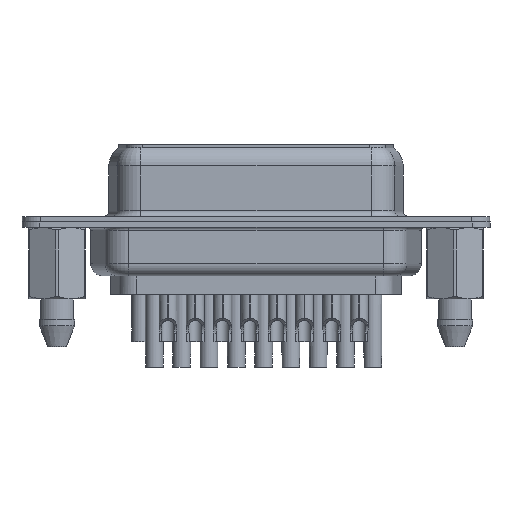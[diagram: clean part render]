
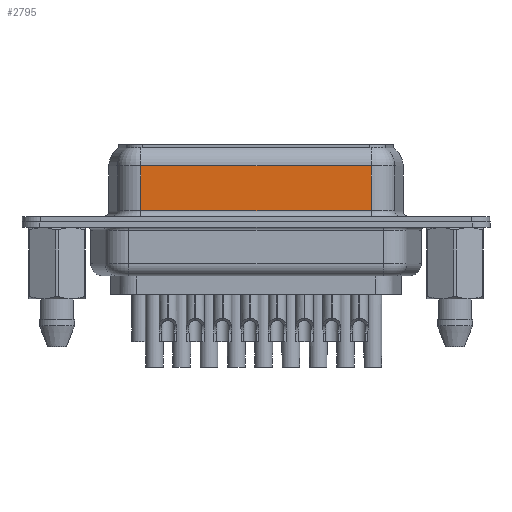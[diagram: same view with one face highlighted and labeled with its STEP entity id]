
A CAD part, front view. The second image highlights one B-rep face of the part: STEP entity #2795.
In plain terms, the highlighted planar face has unit normal (0, -1, 0).
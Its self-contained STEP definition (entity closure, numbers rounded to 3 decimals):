
#271 = EDGE_CURVE ( 'NONE', #7160, #6226, #25439, .T. ) ;
#1505 = ORIENTED_EDGE ( 'NONE', *, *, #20082, .T. ) ;
#2795 = ADVANCED_FACE ( 'NONE', ( #26497 ), #24680, .F. ) ;
#2936 = ORIENTED_EDGE ( 'NONE', *, *, #19702, .F. ) ;
#4737 = VECTOR ( 'NONE', #18753, 1000. ) ;
#5309 = LINE ( 'NONE', #12024, #5910 ) ;
#5910 = VECTOR ( 'NONE', #25761, 1000. ) ;
#5989 = AXIS2_PLACEMENT_3D ( 'NONE', #10464, #28950, #24229 ) ;
#6226 = VERTEX_POINT ( 'NONE', #13155 ) ;
#6380 = CARTESIAN_POINT ( 'NONE',  ( 26.297, -3.95, 4.7 ) ) ;
#6973 = CARTESIAN_POINT ( 'NONE',  ( 26.297, -3.95, 4.7 ) ) ;
#7160 = VERTEX_POINT ( 'NONE', #28946 ) ;
#9443 = CARTESIAN_POINT ( 'NONE',  ( 7.023, -3.95, 4.7 ) ) ;
#10464 = CARTESIAN_POINT ( 'NONE',  ( 26.297, -3.95, 6.45 ) ) ;
#12024 = CARTESIAN_POINT ( 'NONE',  ( 26.297, -3.95, 6.45 ) ) ;
#13155 = CARTESIAN_POINT ( 'NONE',  ( 26.297, -3.95, 0.95 ) ) ;
#14157 = VECTOR ( 'NONE', #20416, 1000. ) ;
#17617 = LINE ( 'NONE', #29498, #29347 ) ;
#18753 = DIRECTION ( 'NONE',  ( -1., 0., 0. ) ) ;
#18808 = ORIENTED_EDGE ( 'NONE', *, *, #271, .T. ) ;
#19702 = EDGE_CURVE ( 'NONE', #21203, #6226, #5309, .T. ) ;
#20082 = EDGE_CURVE ( 'NONE', #20836, #7160, #17617, .T. ) ;
#20416 = DIRECTION ( 'NONE',  ( 1., 0., 0. ) ) ;
#20836 = VERTEX_POINT ( 'NONE', #9443 ) ;
#21135 = EDGE_LOOP ( 'NONE', ( #2936, #24066, #1505, #18808 ) ) ;
#21203 = VERTEX_POINT ( 'NONE', #6380 ) ;
#22871 = CARTESIAN_POINT ( 'NONE',  ( 26.297, -3.95, 0.95 ) ) ;
#24066 = ORIENTED_EDGE ( 'NONE', *, *, #26315, .T. ) ;
#24229 = DIRECTION ( 'NONE',  ( 0., 0., 1. ) ) ;
#24680 = PLANE ( 'NONE',  #5989 ) ;
#25439 = LINE ( 'NONE', #22871, #14157 ) ;
#25761 = DIRECTION ( 'NONE',  ( 0., 0., -1. ) ) ;
#26315 = EDGE_CURVE ( 'NONE', #21203, #20836, #28477, .T. ) ;
#26497 = FACE_OUTER_BOUND ( 'NONE', #21135, .T. ) ;
#28477 = LINE ( 'NONE', #6973, #4737 ) ;
#28946 = CARTESIAN_POINT ( 'NONE',  ( 7.023, -3.95, 0.95 ) ) ;
#28950 = DIRECTION ( 'NONE',  ( 0., 1., 0. ) ) ;
#29038 = DIRECTION ( 'NONE',  ( 0., 0., -1. ) ) ;
#29347 = VECTOR ( 'NONE', #29038, 1000. ) ;
#29498 = CARTESIAN_POINT ( 'NONE',  ( 7.023, -3.95, 6.45 ) ) ;
